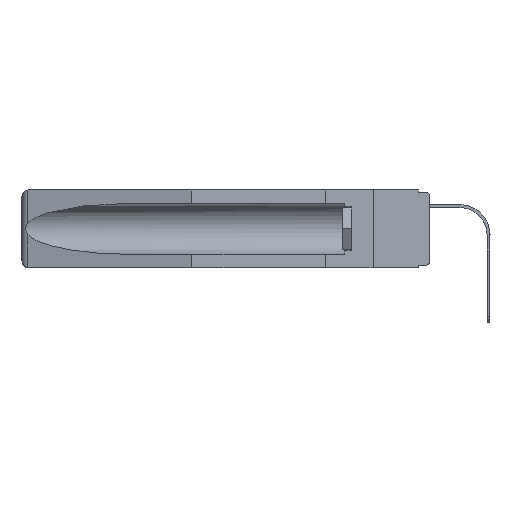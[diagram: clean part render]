
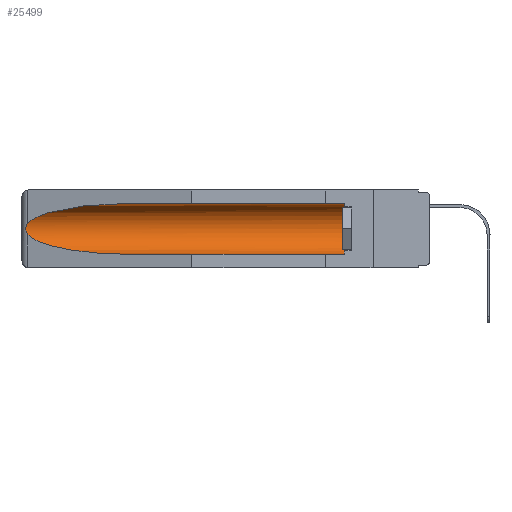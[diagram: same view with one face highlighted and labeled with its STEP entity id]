
A CAD part, left-side view. The second image highlights one B-rep face of the part: STEP entity #25499.
In plain terms, the highlighted cylindrical face has radius 2.857 mm (diameter 5.715 mm), a partial arc.
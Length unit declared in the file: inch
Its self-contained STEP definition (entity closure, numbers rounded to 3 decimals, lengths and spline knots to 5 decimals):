
#1113 = CIRCLE ( 'NONE', #1952, 0.1125 ) ;
#1251 = VERTEX_POINT ( 'NONE', #14787 ) ;
#1325 = VECTOR ( 'NONE', #17021, 39.37008 ) ;
#1952 = AXIS2_PLACEMENT_3D ( 'NONE', #7050, #12577, #24845 ) ;
#2733 = CARTESIAN_POINT ( 'NONE',  ( 0.155, -0.30754, -0.059 ) ) ;
#2742 = CARTESIAN_POINT ( 'NONE',  ( 0.155, 0.126, -0.059 ) ) ;
#2895 = CARTESIAN_POINT ( 'NONE',  ( 0.155, -0.30754, -0.284 ) ) ;
#3022 = DIRECTION ( 'NONE',  ( 0., 0., 1. ) ) ;
#3496 = EDGE_CURVE ( 'NONE', #7882, #5517, #8092, .T. ) ;
#4314 = ORIENTED_EDGE ( 'NONE', *, *, #24466, .T. ) ;
#4407 = CARTESIAN_POINT ( 'NONE',  ( 0.155, 0.126, -0.284 ) ) ;
#4679 = ORIENTED_EDGE ( 'NONE', *, *, #23618, .T. ) ;
#4950 = CARTESIAN_POINT ( 'NONE',  ( 0.21114, 1.30732, -0.059 ) ) ;
#5118 = CARTESIAN_POINT ( 'NONE',  ( 0.2675, 1.53308, -0.16763 ) ) ;
#5131 = ORIENTED_EDGE ( 'NONE', *, *, #9723, .F. ) ;
#5363 = VERTEX_POINT ( 'NONE', #8363 ) ;
#5517 = VERTEX_POINT ( 'NONE', #9646 ) ;
#5760 = VERTEX_POINT ( 'NONE', #2742 ) ;
#6908 = VECTOR ( 'NONE', #18857, 39.37008 ) ;
#7050 = CARTESIAN_POINT ( 'NONE',  ( 0.155, 0.126, -0.1715 ) ) ;
#7124 = CARTESIAN_POINT ( 'NONE',  ( 0.26654, 1.53092, -0.15636 ) ) ;
#7146 = CARTESIAN_POINT ( 'NONE',  ( 0.155, -0.30754, -0.1715 ) ) ;
#7361 = VERTEX_POINT ( 'NONE', #4407 ) ;
#7882 = VERTEX_POINT ( 'NONE', #10245 ) ;
#8092 =( BOUNDED_CURVE ( )  B_SPLINE_CURVE ( 3, ( #15179, #23196, #13181, #25308 ),
 .UNSPECIFIED., .F., .T. ) 
 B_SPLINE_CURVE_WITH_KNOTS ( ( 4, 4 ),
 ( 0.1948, 1.5708 ),
 .UNSPECIFIED. ) 
 CURVE ( )  GEOMETRIC_REPRESENTATION_ITEM ( )  RATIONAL_B_SPLINE_CURVE ( ( 1., 0.848, 0.848, 1. ) ) 
 REPRESENTATION_ITEM ( '' )  );
#8162 = CARTESIAN_POINT ( 'NONE',  ( 0.26655, 1.53094, -0.18657 ) ) ;
#8210 = B_SPLINE_CURVE_WITH_KNOTS ( 'NONE', 3,
 ( #25178, #17139, #7124, #15174, #5118, #13176, #21223, #8162, #15701, #16082 ),
 .UNSPECIFIED., .F., .F.,
 ( 4, 2, 2, 2, 4 ),
 ( 0., 0.00029, 0.00058, 0.00087, 0.00117 ),
 .UNSPECIFIED. ) ;
#8363 = CARTESIAN_POINT ( 'NONE',  ( 0.155, 1.07973, -0.059 ) ) ;
#9365 = ORIENTED_EDGE ( 'NONE', *, *, #11572, .T. ) ;
#9646 = CARTESIAN_POINT ( 'NONE',  ( 0.155, 1.07973, -0.284 ) ) ;
#9723 = EDGE_CURVE ( 'NONE', #7361, #5517, #22815, .T. ) ;
#10245 = CARTESIAN_POINT ( 'NONE',  ( 0.26537, 1.52718, -0.19328 ) ) ;
#11572 = EDGE_CURVE ( 'NONE', #1251, #7882, #8210, .T. ) ;
#12577 = DIRECTION ( 'NONE',  ( 0., -1., 0. ) ) ;
#12765 = LINE ( 'NONE', #2733, #6908 ) ;
#13007 = CARTESIAN_POINT ( 'NONE',  ( 0.26537, 1.52718, -0.14972 ) ) ;
#13176 = CARTESIAN_POINT ( 'NONE',  ( 0.2675, 1.53308, -0.17534 ) ) ;
#13181 = CARTESIAN_POINT ( 'NONE',  ( 0.21114, 1.30732, -0.284 ) ) ;
#13483 =( BOUNDED_CURVE ( )  B_SPLINE_CURVE ( 3, ( #23150, #4950, #14994, #13007 ),
 .UNSPECIFIED., .F., .T. ) 
 B_SPLINE_CURVE_WITH_KNOTS ( ( 4, 4 ),
 ( 4.71239, 6.08839 ),
 .UNSPECIFIED. ) 
 CURVE ( )  GEOMETRIC_REPRESENTATION_ITEM ( )  RATIONAL_B_SPLINE_CURVE ( ( 1., 0.848, 0.848, 1. ) ) 
 REPRESENTATION_ITEM ( '' )  );
#14344 = ORIENTED_EDGE ( 'NONE', *, *, #3496, .T. ) ;
#14787 = CARTESIAN_POINT ( 'NONE',  ( 0.26537, 1.52718, -0.14972 ) ) ;
#14994 = CARTESIAN_POINT ( 'NONE',  ( 0.25451, 1.48313, -0.09465 ) ) ;
#15174 = CARTESIAN_POINT ( 'NONE',  ( 0.2673, 1.5327, -0.16383 ) ) ;
#15179 = CARTESIAN_POINT ( 'NONE',  ( 0.26537, 1.52718, -0.19328 ) ) ;
#15701 = CARTESIAN_POINT ( 'NONE',  ( 0.26597, 1.5296, -0.19026 ) ) ;
#16082 = CARTESIAN_POINT ( 'NONE',  ( 0.26537, 1.52718, -0.19328 ) ) ;
#16905 = DIRECTION ( 'NONE',  ( 0., 1., 0. ) ) ;
#17021 = DIRECTION ( 'NONE',  ( 0., 1., 0. ) ) ;
#17026 = CYLINDRICAL_SURFACE ( 'NONE', #25632, 0.1125 ) ;
#17139 = CARTESIAN_POINT ( 'NONE',  ( 0.26597, 1.52961, -0.15275 ) ) ;
#17801 = EDGE_CURVE ( 'NONE', #5760, #5363, #12765, .T. ) ;
#18161 = ORIENTED_EDGE ( 'NONE', *, *, #17801, .T. ) ;
#18857 = DIRECTION ( 'NONE',  ( 0., 1., 0. ) ) ;
#20483 = EDGE_LOOP ( 'NONE', ( #4314, #9365, #14344, #5131, #4679, #18161 ) ) ;
#21223 = CARTESIAN_POINT ( 'NONE',  ( 0.2673, 1.53269, -0.17917 ) ) ;
#22815 = LINE ( 'NONE', #2895, #1325 ) ;
#23150 = CARTESIAN_POINT ( 'NONE',  ( 0.155, 1.07973, -0.059 ) ) ;
#23196 = CARTESIAN_POINT ( 'NONE',  ( 0.25451, 1.48313, -0.24835 ) ) ;
#23212 = FACE_OUTER_BOUND ( 'NONE', #20483, .T. ) ;
#23618 = EDGE_CURVE ( 'NONE', #7361, #5760, #1113, .T. ) ;
#24466 = EDGE_CURVE ( 'NONE', #5363, #1251, #13483, .T. ) ;
#24845 = DIRECTION ( 'NONE',  ( 0., 0., 1. ) ) ;
#25178 = CARTESIAN_POINT ( 'NONE',  ( 0.26537, 1.52718, -0.14972 ) ) ;
#25308 = CARTESIAN_POINT ( 'NONE',  ( 0.155, 1.07973, -0.284 ) ) ;
#25499 = ADVANCED_FACE ( 'NONE', ( #23212 ), #17026, .F. ) ;
#25632 = AXIS2_PLACEMENT_3D ( 'NONE', #7146, #16905, #3022 ) ;
